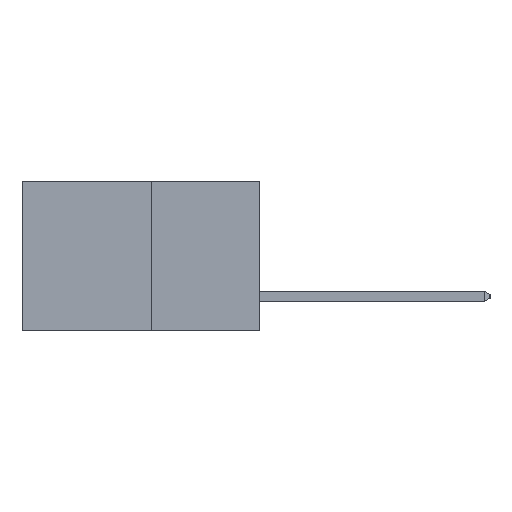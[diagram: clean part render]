
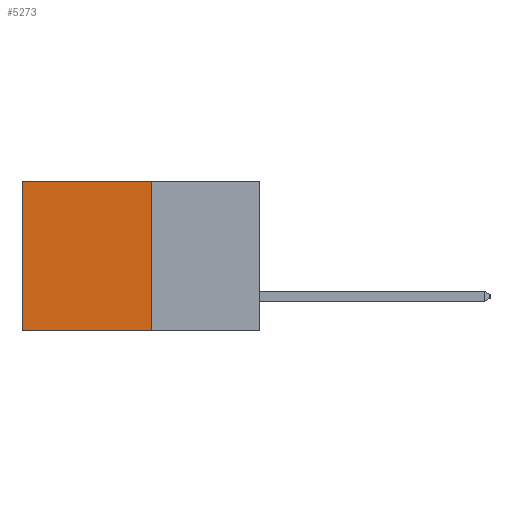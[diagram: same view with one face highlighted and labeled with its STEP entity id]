
A CAD part, left-side view. The second image highlights one B-rep face of the part: STEP entity #5273.
In plain terms, the highlighted planar face has unit normal (-1, 0, 0).
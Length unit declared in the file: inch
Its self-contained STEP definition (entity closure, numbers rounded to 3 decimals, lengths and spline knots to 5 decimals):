
#541 = CARTESIAN_POINT ( 'NONE',  ( 0.277, 0.27, -0.37 ) ) ;
#657 = PLANE ( 'NONE',  #7342 ) ;
#714 = DIRECTION ( 'NONE',  ( 0., 0., -1. ) ) ;
#734 = DIRECTION ( 'NONE',  ( 1., 0., 0. ) ) ;
#893 = EDGE_CURVE ( 'NONE', #8864, #9742, #3506, .T. ) ;
#1410 = CARTESIAN_POINT ( 'NONE',  ( 0.277, 0.27, -0.37 ) ) ;
#1618 = FACE_OUTER_BOUND ( 'NONE', #5339, .T. ) ;
#1779 = LINE ( 'NONE', #5868, #11537 ) ;
#3506 = LINE ( 'NONE', #9524, #9177 ) ;
#3576 = EDGE_CURVE ( 'NONE', #4767, #7093, #10846, .T. ) ;
#3731 = CARTESIAN_POINT ( 'NONE',  ( 0.277, 0.59, -0.37 ) ) ;
#3884 = CARTESIAN_POINT ( 'NONE',  ( 0.277, 0.59, 0. ) ) ;
#4176 = EDGE_CURVE ( 'NONE', #8864, #4767, #1779, .T. ) ;
#4767 = VERTEX_POINT ( 'NONE', #3884 ) ;
#5190 = ORIENTED_EDGE ( 'NONE', *, *, #3576, .T. ) ;
#5273 = ADVANCED_FACE ( 'NONE', ( #1618 ), #657, .F. ) ;
#5283 = ORIENTED_EDGE ( 'NONE', *, *, #10903, .F. ) ;
#5339 = EDGE_LOOP ( 'NONE', ( #5190, #5283, #6092, #6333 ) ) ;
#5868 = CARTESIAN_POINT ( 'NONE',  ( 0.277, 0.27, 0. ) ) ;
#6092 = ORIENTED_EDGE ( 'NONE', *, *, #893, .F. ) ;
#6231 = CARTESIAN_POINT ( 'NONE',  ( 0.277, 0.27, -0.37 ) ) ;
#6333 = ORIENTED_EDGE ( 'NONE', *, *, #4176, .T. ) ;
#7093 = VERTEX_POINT ( 'NONE', #3731 ) ;
#7119 = DIRECTION ( 'NONE',  ( 0., 1., 0. ) ) ;
#7342 = AXIS2_PLACEMENT_3D ( 'NONE', #541, #734, #714 ) ;
#8398 = VECTOR ( 'NONE', #8860, 39.37008 ) ;
#8823 = CARTESIAN_POINT ( 'NONE',  ( 0.277, 0.59, -0.37 ) ) ;
#8860 = DIRECTION ( 'NONE',  ( 0., 0., -1. ) ) ;
#8864 = VERTEX_POINT ( 'NONE', #10380 ) ;
#8931 = VECTOR ( 'NONE', #9038, 39.37008 ) ;
#9038 = DIRECTION ( 'NONE',  ( 0., 1., 0. ) ) ;
#9146 = DIRECTION ( 'NONE',  ( 0., 0., -1. ) ) ;
#9177 = VECTOR ( 'NONE', #9146, 39.37008 ) ;
#9524 = CARTESIAN_POINT ( 'NONE',  ( 0.277, 0.27, -0.37 ) ) ;
#9742 = VERTEX_POINT ( 'NONE', #1410 ) ;
#10380 = CARTESIAN_POINT ( 'NONE',  ( 0.277, 0.27, 0. ) ) ;
#10846 = LINE ( 'NONE', #8823, #8398 ) ;
#10903 = EDGE_CURVE ( 'NONE', #9742, #7093, #11366, .T. ) ;
#11366 = LINE ( 'NONE', #6231, #8931 ) ;
#11537 = VECTOR ( 'NONE', #7119, 39.37008 ) ;
